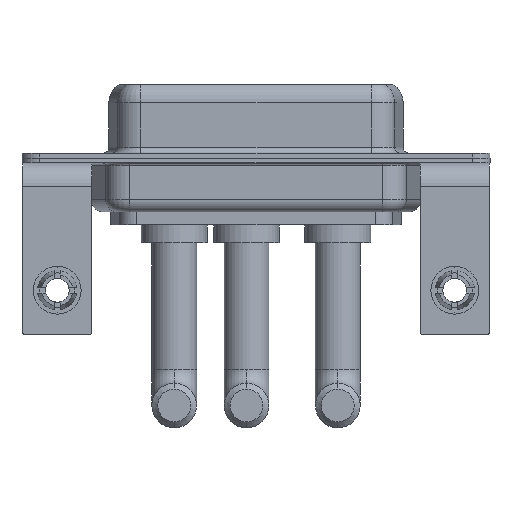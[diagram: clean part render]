
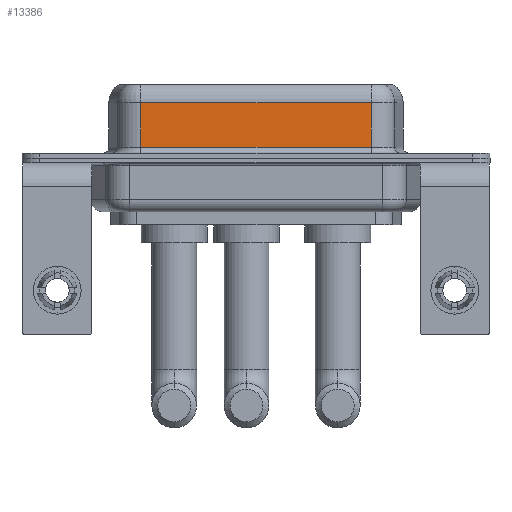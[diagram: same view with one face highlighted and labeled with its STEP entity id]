
A CAD part, front view. The second image highlights one B-rep face of the part: STEP entity #13386.
In plain terms, the highlighted planar face has unit normal (0, -1, 0).
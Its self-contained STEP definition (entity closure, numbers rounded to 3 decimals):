
#103 = VERTEX_POINT ( 'NONE', #12012 ) ;
#282 = VERTEX_POINT ( 'NONE', #4244 ) ;
#501 = CARTESIAN_POINT ( 'NONE',  ( 26.287, -3.95, 0.9 ) ) ;
#639 = VECTOR ( 'NONE', #10060, 1000. ) ;
#1247 = ORIENTED_EDGE ( 'NONE', *, *, #10099, .F. ) ;
#1274 = DIRECTION ( 'NONE',  ( 0., 0., 1. ) ) ;
#1943 = VERTEX_POINT ( 'NONE', #15532 ) ;
#2239 = LINE ( 'NONE', #12321, #12620 ) ;
#2508 = PLANE ( 'NONE',  #10881 ) ;
#4244 = CARTESIAN_POINT ( 'NONE',  ( 7.013, -3.95, 0.9 ) ) ;
#4595 = EDGE_CURVE ( 'NONE', #15688, #103, #12910, .T. ) ;
#4741 = DIRECTION ( 'NONE',  ( 0., 0., -1. ) ) ;
#4888 = FACE_OUTER_BOUND ( 'NONE', #7602, .T. ) ;
#6119 = ORIENTED_EDGE ( 'NONE', *, *, #8504, .T. ) ;
#6967 = ORIENTED_EDGE ( 'NONE', *, *, #8703, .T. ) ;
#7591 = CARTESIAN_POINT ( 'NONE',  ( 26.287, -3.95, 4.65 ) ) ;
#7602 = EDGE_LOOP ( 'NONE', ( #1247, #9928, #6967, #6119 ) ) ;
#8504 = EDGE_CURVE ( 'NONE', #282, #1943, #11678, .T. ) ;
#8703 = EDGE_CURVE ( 'NONE', #103, #282, #2239, .T. ) ;
#9702 = LINE ( 'NONE', #13452, #10311 ) ;
#9928 = ORIENTED_EDGE ( 'NONE', *, *, #4595, .T. ) ;
#10060 = DIRECTION ( 'NONE',  ( 1., 0., 0. ) ) ;
#10099 = EDGE_CURVE ( 'NONE', #15688, #1943, #9702, .T. ) ;
#10311 = VECTOR ( 'NONE', #4741, 1000. ) ;
#10388 = DIRECTION ( 'NONE',  ( -1., 0., 0. ) ) ;
#10544 = CARTESIAN_POINT ( 'NONE',  ( 26.287, -3.95, 4.65 ) ) ;
#10881 = AXIS2_PLACEMENT_3D ( 'NONE', #12432, #12270, #1274 ) ;
#11678 = LINE ( 'NONE', #501, #639 ) ;
#12012 = CARTESIAN_POINT ( 'NONE',  ( 7.013, -3.95, 4.65 ) ) ;
#12270 = DIRECTION ( 'NONE',  ( 0., 1., 0. ) ) ;
#12321 = CARTESIAN_POINT ( 'NONE',  ( 7.013, -3.95, 6.4 ) ) ;
#12432 = CARTESIAN_POINT ( 'NONE',  ( 26.287, -3.95, 6.4 ) ) ;
#12620 = VECTOR ( 'NONE', #13569, 1000. ) ;
#12910 = LINE ( 'NONE', #10544, #15469 ) ;
#13386 = ADVANCED_FACE ( 'NONE', ( #4888 ), #2508, .F. ) ;
#13452 = CARTESIAN_POINT ( 'NONE',  ( 26.287, -3.95, 6.4 ) ) ;
#13569 = DIRECTION ( 'NONE',  ( 0., 0., -1. ) ) ;
#15469 = VECTOR ( 'NONE', #10388, 1000. ) ;
#15532 = CARTESIAN_POINT ( 'NONE',  ( 26.287, -3.95, 0.9 ) ) ;
#15688 = VERTEX_POINT ( 'NONE', #7591 ) ;
